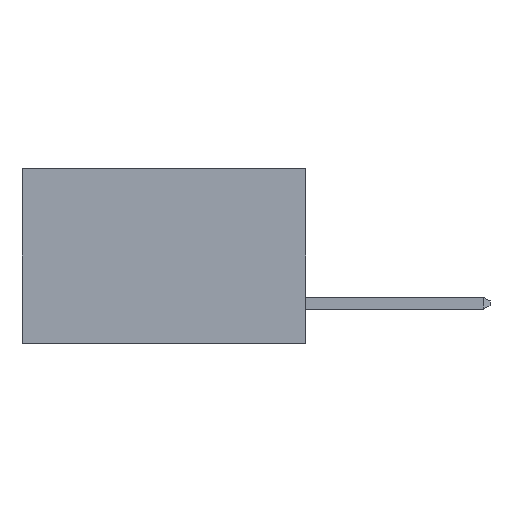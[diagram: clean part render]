
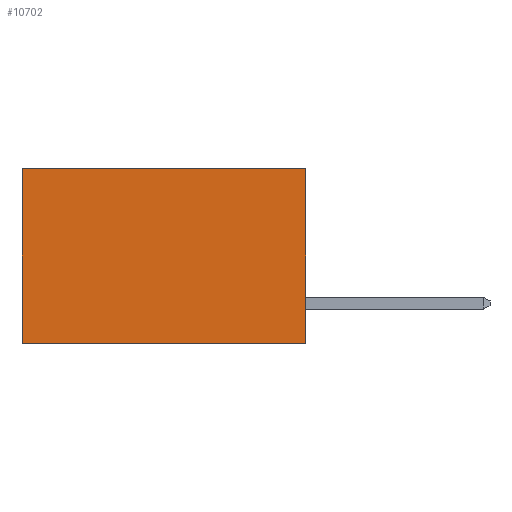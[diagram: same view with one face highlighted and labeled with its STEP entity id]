
A CAD part, left-side view. The second image highlights one B-rep face of the part: STEP entity #10702.
In plain terms, the highlighted planar face has unit normal (-1, 0, 0).
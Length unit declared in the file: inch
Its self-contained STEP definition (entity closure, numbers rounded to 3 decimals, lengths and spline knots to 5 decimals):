
#40 = EDGE_CURVE ( 'NONE', #7010, #10185, #7144, .T. ) ;
#761 = EDGE_CURVE ( 'NONE', #8240, #7010, #15116, .T. ) ;
#1177 = EDGE_CURVE ( 'NONE', #10142, #10185, #8307, .T. ) ;
#1887 = CARTESIAN_POINT ( 'NONE',  ( 0.298, 0., 0. ) ) ;
#2676 = CARTESIAN_POINT ( 'NONE',  ( 0.298, 0.6, -0.37 ) ) ;
#3848 = VECTOR ( 'NONE', #10116, 39.37008 ) ;
#4817 = VECTOR ( 'NONE', #8054, 39.37008 ) ;
#5248 = PLANE ( 'NONE',  #12004 ) ;
#5882 = CARTESIAN_POINT ( 'NONE',  ( 0.298, 0., 0. ) ) ;
#7010 = VERTEX_POINT ( 'NONE', #7547 ) ;
#7144 = LINE ( 'NONE', #11207, #3848 ) ;
#7547 = CARTESIAN_POINT ( 'NONE',  ( 0.298, 0., -0.37 ) ) ;
#7619 = DIRECTION ( 'NONE',  ( 0., 0., -1. ) ) ;
#7950 = CARTESIAN_POINT ( 'NONE',  ( 0.298, 0.6, 0. ) ) ;
#8054 = DIRECTION ( 'NONE',  ( 0., 0., -1. ) ) ;
#8240 = VERTEX_POINT ( 'NONE', #12676 ) ;
#8307 = LINE ( 'NONE', #7950, #4817 ) ;
#8479 = DIRECTION ( 'NONE',  ( 0., 0., -1. ) ) ;
#10116 = DIRECTION ( 'NONE',  ( 0., 1., 0. ) ) ;
#10142 = VERTEX_POINT ( 'NONE', #15443 ) ;
#10185 = VERTEX_POINT ( 'NONE', #2676 ) ;
#10581 = VECTOR ( 'NONE', #14859, 39.37008 ) ;
#10702 = ADVANCED_FACE ( 'NONE', ( #14728 ), #5248, .F. ) ;
#11112 = EDGE_CURVE ( 'NONE', #8240, #10142, #13193, .T. ) ;
#11207 = CARTESIAN_POINT ( 'NONE',  ( 0.298, 0., -0.37 ) ) ;
#12004 = AXIS2_PLACEMENT_3D ( 'NONE', #13225, #14318, #7619 ) ;
#12204 = VECTOR ( 'NONE', #8479, 39.37008 ) ;
#12676 = CARTESIAN_POINT ( 'NONE',  ( 0.298, 0., 0. ) ) ;
#13023 = ORIENTED_EDGE ( 'NONE', *, *, #11112, .T. ) ;
#13193 = LINE ( 'NONE', #5882, #10581 ) ;
#13225 = CARTESIAN_POINT ( 'NONE',  ( 0.298, 0., 0. ) ) ;
#13296 = ORIENTED_EDGE ( 'NONE', *, *, #40, .F. ) ;
#13416 = ORIENTED_EDGE ( 'NONE', *, *, #761, .F. ) ;
#13483 = ORIENTED_EDGE ( 'NONE', *, *, #1177, .T. ) ;
#13540 = EDGE_LOOP ( 'NONE', ( #13483, #13296, #13416, #13023 ) ) ;
#14318 = DIRECTION ( 'NONE',  ( 1., 0., 0. ) ) ;
#14728 = FACE_OUTER_BOUND ( 'NONE', #13540, .T. ) ;
#14859 = DIRECTION ( 'NONE',  ( 0., 1., 0. ) ) ;
#15116 = LINE ( 'NONE', #1887, #12204 ) ;
#15443 = CARTESIAN_POINT ( 'NONE',  ( 0.298, 0.6, 0. ) ) ;
